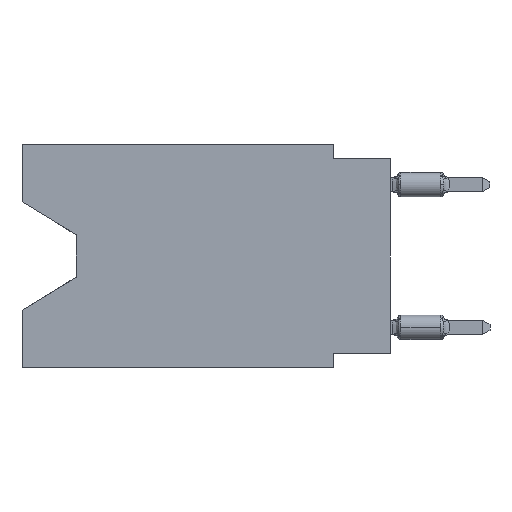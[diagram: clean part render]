
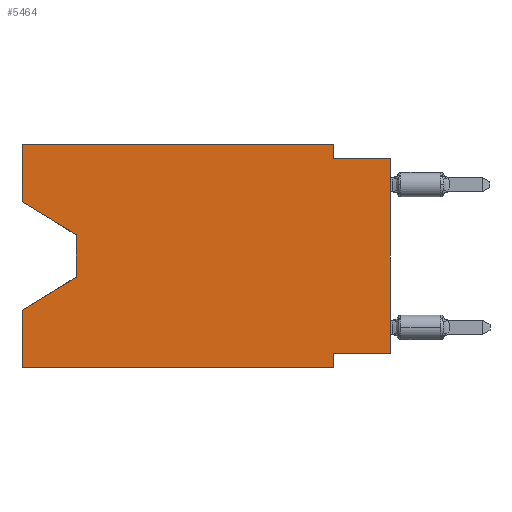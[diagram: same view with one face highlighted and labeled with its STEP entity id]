
A CAD part, left-side view. The second image highlights one B-rep face of the part: STEP entity #5464.
In plain terms, the highlighted planar face has unit normal (-1, 0, 0).
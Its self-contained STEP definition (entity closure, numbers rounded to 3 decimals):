
#119 = EDGE_CURVE ( 'NONE', #7128, #1728, #4898, .T. ) ;
#229 = ORIENTED_EDGE ( 'NONE', *, *, #1434, .F. ) ;
#289 = DIRECTION ( 'NONE',  ( 0., 0., 1. ) ) ;
#296 = VECTOR ( 'NONE', #11356, 1000. ) ;
#384 = CARTESIAN_POINT ( 'NONE',  ( 0., 0., 0. ) ) ;
#391 = CARTESIAN_POINT ( 'NONE',  ( 0., 13.97, -5.893 ) ) ;
#460 = VECTOR ( 'NONE', #289, 1000. ) ;
#462 = CARTESIAN_POINT ( 'NONE',  ( 0., 13.97, -4.013 ) ) ;
#531 = CARTESIAN_POINT ( 'NONE',  ( 0., 2.54, -9.271 ) ) ;
#635 = VECTOR ( 'NONE', #9536, 1000. ) ;
#649 = EDGE_CURVE ( 'NONE', #12605, #5453, #1129, .T. ) ;
#728 = VECTOR ( 'NONE', #11439, 1000. ) ;
#910 = LINE ( 'NONE', #12127, #11590 ) ;
#1129 = LINE ( 'NONE', #3951, #5370 ) ;
#1160 = AXIS2_PLACEMENT_3D ( 'NONE', #12660, #4709, #1763 ) ;
#1210 = EDGE_CURVE ( 'NONE', #5635, #8447, #2222, .T. ) ;
#1370 = LINE ( 'NONE', #384, #9492 ) ;
#1434 = EDGE_CURVE ( 'NONE', #8786, #6031, #910, .T. ) ;
#1728 = VERTEX_POINT ( 'NONE', #11855 ) ;
#1763 = DIRECTION ( 'NONE',  ( 0., 0., -1. ) ) ;
#1895 = DIRECTION ( 'NONE',  ( 0., 1., 0. ) ) ;
#1907 = CARTESIAN_POINT ( 'NONE',  ( 0., 16.383, -2.546 ) ) ;
#2222 = LINE ( 'NONE', #391, #296 ) ;
#2225 = EDGE_CURVE ( 'NONE', #3946, #7128, #2369, .T. ) ;
#2369 = LINE ( 'NONE', #12420, #635 ) ;
#2388 = CARTESIAN_POINT ( 'NONE',  ( 0., 13.97, -5.893 ) ) ;
#2391 = CARTESIAN_POINT ( 'NONE',  ( 0., 2.54, -9.906 ) ) ;
#2430 = CARTESIAN_POINT ( 'NONE',  ( 0., 16.383, -9.906 ) ) ;
#2563 = LINE ( 'NONE', #2430, #3653 ) ;
#2616 = DIRECTION ( 'NONE',  ( 0., -1., 0. ) ) ;
#2649 = EDGE_CURVE ( 'NONE', #3341, #3946, #12656, .T. ) ;
#2737 = DIRECTION ( 'NONE',  ( 0., -1., 0. ) ) ;
#2951 = VERTEX_POINT ( 'NONE', #4287 ) ;
#3260 = DIRECTION ( 'NONE',  ( 0., 0., 1. ) ) ;
#3276 = DIRECTION ( 'NONE',  ( 0., -1., 0. ) ) ;
#3341 = VERTEX_POINT ( 'NONE', #11183 ) ;
#3515 = ORIENTED_EDGE ( 'NONE', *, *, #12049, .F. ) ;
#3653 = VECTOR ( 'NONE', #3276, 1000. ) ;
#3669 = ORIENTED_EDGE ( 'NONE', *, *, #10180, .F. ) ;
#3814 = ORIENTED_EDGE ( 'NONE', *, *, #649, .T. ) ;
#3858 = LINE ( 'NONE', #5788, #10821 ) ;
#3946 = VERTEX_POINT ( 'NONE', #10774 ) ;
#3951 = CARTESIAN_POINT ( 'NONE',  ( 0., 16.383, -2.546 ) ) ;
#4245 = ORIENTED_EDGE ( 'NONE', *, *, #7741, .T. ) ;
#4287 = CARTESIAN_POINT ( 'NONE',  ( 0., 16.383, -9.906 ) ) ;
#4709 = DIRECTION ( 'NONE',  ( 1., 0., 0. ) ) ;
#4889 = ORIENTED_EDGE ( 'NONE', *, *, #7725, .T. ) ;
#4898 = LINE ( 'NONE', #7916, #12697 ) ;
#5033 = VECTOR ( 'NONE', #2616, 1000. ) ;
#5086 = EDGE_CURVE ( 'NONE', #6031, #5702, #3858, .T. ) ;
#5370 = VECTOR ( 'NONE', #9197, 1000. ) ;
#5453 = VERTEX_POINT ( 'NONE', #11614 ) ;
#5464 = ADVANCED_FACE ( 'NONE', ( #6744 ), #10763, .F. ) ;
#5635 = VERTEX_POINT ( 'NONE', #2388 ) ;
#5683 = CARTESIAN_POINT ( 'NONE',  ( 0., 2.54, -0.635 ) ) ;
#5702 = VERTEX_POINT ( 'NONE', #2391 ) ;
#5788 = CARTESIAN_POINT ( 'NONE',  ( 0., 2.54, -9.906 ) ) ;
#6031 = VERTEX_POINT ( 'NONE', #531 ) ;
#6151 = ORIENTED_EDGE ( 'NONE', *, *, #1210, .T. ) ;
#6258 = LINE ( 'NONE', #10264, #460 ) ;
#6293 = CARTESIAN_POINT ( 'NONE',  ( 0., 16.383, 0. ) ) ;
#6347 = VECTOR ( 'NONE', #10086, 1000. ) ;
#6744 = FACE_OUTER_BOUND ( 'NONE', #6978, .T. ) ;
#6978 = EDGE_LOOP ( 'NONE', ( #3814, #4889, #6151, #3669, #4245, #12945, #229, #12906, #9317, #11844, #10335, #3515 ) ) ;
#7128 = VERTEX_POINT ( 'NONE', #5683 ) ;
#7241 = CARTESIAN_POINT ( 'NONE',  ( 0., 16.383, -7.36 ) ) ;
#7725 = EDGE_CURVE ( 'NONE', #5453, #5635, #11561, .T. ) ;
#7741 = EDGE_CURVE ( 'NONE', #2951, #5702, #2563, .T. ) ;
#7828 = CARTESIAN_POINT ( 'NONE',  ( 0., 0., -9.271 ) ) ;
#7916 = CARTESIAN_POINT ( 'NONE',  ( 0., 0., -0.635 ) ) ;
#8447 = VERTEX_POINT ( 'NONE', #7241 ) ;
#8786 = VERTEX_POINT ( 'NONE', #7828 ) ;
#8851 = CARTESIAN_POINT ( 'NONE',  ( 0., 16.383, 0. ) ) ;
#8978 = LINE ( 'NONE', #8851, #6347 ) ;
#9197 = DIRECTION ( 'NONE',  ( 0., -0.855, -0.519 ) ) ;
#9317 = ORIENTED_EDGE ( 'NONE', *, *, #119, .F. ) ;
#9492 = VECTOR ( 'NONE', #3260, 1000. ) ;
#9536 = DIRECTION ( 'NONE',  ( 0., 0., -1. ) ) ;
#9917 = EDGE_CURVE ( 'NONE', #8786, #1728, #1370, .T. ) ;
#10086 = DIRECTION ( 'NONE',  ( 0., 0., 1. ) ) ;
#10180 = EDGE_CURVE ( 'NONE', #2951, #8447, #8978, .T. ) ;
#10264 = CARTESIAN_POINT ( 'NONE',  ( 0., 16.383, 0. ) ) ;
#10335 = ORIENTED_EDGE ( 'NONE', *, *, #2649, .F. ) ;
#10763 = PLANE ( 'NONE',  #1160 ) ;
#10774 = CARTESIAN_POINT ( 'NONE',  ( 0., 2.54, 0. ) ) ;
#10821 = VECTOR ( 'NONE', #11626, 1000. ) ;
#11183 = CARTESIAN_POINT ( 'NONE',  ( 0., 16.383, 0. ) ) ;
#11356 = DIRECTION ( 'NONE',  ( 0., 0.855, -0.519 ) ) ;
#11439 = DIRECTION ( 'NONE',  ( 0., 0., -1. ) ) ;
#11561 = LINE ( 'NONE', #462, #728 ) ;
#11590 = VECTOR ( 'NONE', #1895, 1000. ) ;
#11614 = CARTESIAN_POINT ( 'NONE',  ( 0., 13.97, -4.013 ) ) ;
#11626 = DIRECTION ( 'NONE',  ( 0., 0., -1. ) ) ;
#11844 = ORIENTED_EDGE ( 'NONE', *, *, #2225, .F. ) ;
#11855 = CARTESIAN_POINT ( 'NONE',  ( 0., 0., -0.635 ) ) ;
#12049 = EDGE_CURVE ( 'NONE', #12605, #3341, #6258, .T. ) ;
#12127 = CARTESIAN_POINT ( 'NONE',  ( 0., 0., -9.271 ) ) ;
#12420 = CARTESIAN_POINT ( 'NONE',  ( 0., 2.54, 0. ) ) ;
#12605 = VERTEX_POINT ( 'NONE', #1907 ) ;
#12656 = LINE ( 'NONE', #6293, #5033 ) ;
#12660 = CARTESIAN_POINT ( 'NONE',  ( 0., 16.383, 0. ) ) ;
#12697 = VECTOR ( 'NONE', #2737, 1000. ) ;
#12906 = ORIENTED_EDGE ( 'NONE', *, *, #9917, .T. ) ;
#12945 = ORIENTED_EDGE ( 'NONE', *, *, #5086, .F. ) ;
